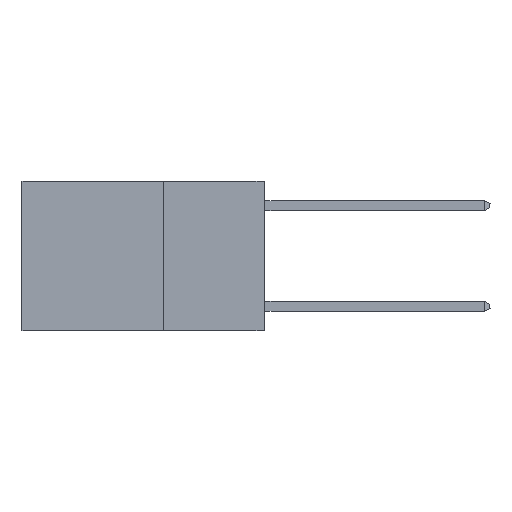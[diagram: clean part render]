
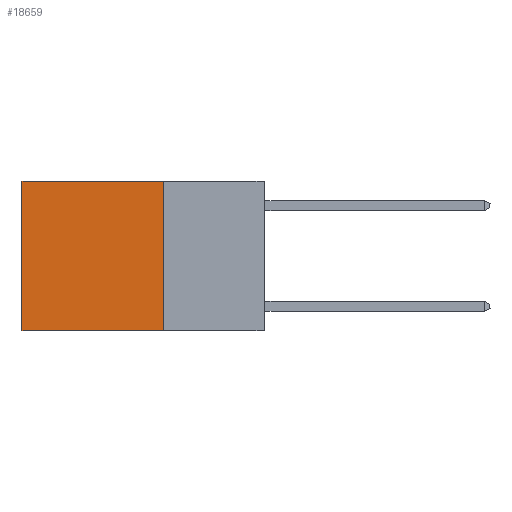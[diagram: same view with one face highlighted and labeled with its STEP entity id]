
A CAD part, left-side view. The second image highlights one B-rep face of the part: STEP entity #18659.
In plain terms, the highlighted planar face has unit normal (-1, 0, 0).
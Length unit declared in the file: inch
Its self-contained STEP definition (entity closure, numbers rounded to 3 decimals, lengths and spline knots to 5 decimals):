
#725 = EDGE_CURVE ( 'NONE', #21521, #13456, #14026, .T. ) ;
#916 = VERTEX_POINT ( 'NONE', #14855 ) ;
#1627 = EDGE_LOOP ( 'NONE', ( #5259, #19021, #6137, #10518 ) ) ;
#2569 = CARTESIAN_POINT ( 'NONE',  ( 0.2625, 0.6, -0.37 ) ) ;
#2905 = VERTEX_POINT ( 'NONE', #13208 ) ;
#4816 = DIRECTION ( 'NONE',  ( 0., 1., 0. ) ) ;
#4976 = LINE ( 'NONE', #14594, #24013 ) ;
#5259 = ORIENTED_EDGE ( 'NONE', *, *, #13820, .T. ) ;
#6137 = ORIENTED_EDGE ( 'NONE', *, *, #24850, .F. ) ;
#6999 = CARTESIAN_POINT ( 'NONE',  ( 0.2625, 0.25, 0. ) ) ;
#8697 = VECTOR ( 'NONE', #19912, 39.37008 ) ;
#8944 = VECTOR ( 'NONE', #17991, 39.37008 ) ;
#9047 = DIRECTION ( 'NONE',  ( 0., 0., -1. ) ) ;
#10130 = LINE ( 'NONE', #14124, #8944 ) ;
#10192 = LINE ( 'NONE', #18303, #11841 ) ;
#10518 = ORIENTED_EDGE ( 'NONE', *, *, #12623, .T. ) ;
#10590 = DIRECTION ( 'NONE',  ( 1., 0., 0. ) ) ;
#11841 = VECTOR ( 'NONE', #4816, 39.37008 ) ;
#12623 = EDGE_CURVE ( 'NONE', #2905, #916, #10192, .T. ) ;
#13208 = CARTESIAN_POINT ( 'NONE',  ( 0.2625, 0.25, 0. ) ) ;
#13456 = VERTEX_POINT ( 'NONE', #2569 ) ;
#13820 = EDGE_CURVE ( 'NONE', #916, #13456, #4976, .T. ) ;
#14026 = LINE ( 'NONE', #21865, #8697 ) ;
#14030 = CARTESIAN_POINT ( 'NONE',  ( 0.2625, 0.25, -0.37 ) ) ;
#14124 = CARTESIAN_POINT ( 'NONE',  ( 0.2625, 0.25, 0. ) ) ;
#14594 = CARTESIAN_POINT ( 'NONE',  ( 0.2625, 0.6, 0. ) ) ;
#14855 = CARTESIAN_POINT ( 'NONE',  ( 0.2625, 0.6, 0. ) ) ;
#17499 = AXIS2_PLACEMENT_3D ( 'NONE', #6999, #10590, #9047 ) ;
#17991 = DIRECTION ( 'NONE',  ( 0., 0., -1. ) ) ;
#18303 = CARTESIAN_POINT ( 'NONE',  ( 0.2625, 0.25, 0. ) ) ;
#18659 = ADVANCED_FACE ( 'NONE', ( #22566 ), #22797, .F. ) ;
#19021 = ORIENTED_EDGE ( 'NONE', *, *, #725, .F. ) ;
#19912 = DIRECTION ( 'NONE',  ( 0., 1., 0. ) ) ;
#21521 = VERTEX_POINT ( 'NONE', #14030 ) ;
#21865 = CARTESIAN_POINT ( 'NONE',  ( 0.2625, 0.25, -0.37 ) ) ;
#22566 = FACE_OUTER_BOUND ( 'NONE', #1627, .T. ) ;
#22797 = PLANE ( 'NONE',  #17499 ) ;
#24013 = VECTOR ( 'NONE', #24467, 39.37008 ) ;
#24467 = DIRECTION ( 'NONE',  ( 0., 0., -1. ) ) ;
#24850 = EDGE_CURVE ( 'NONE', #2905, #21521, #10130, .T. ) ;
